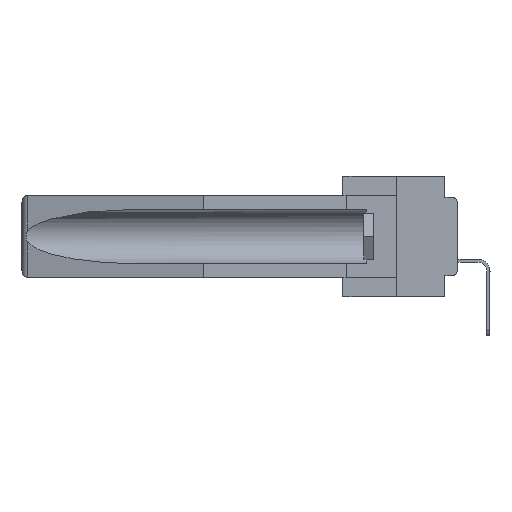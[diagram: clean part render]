
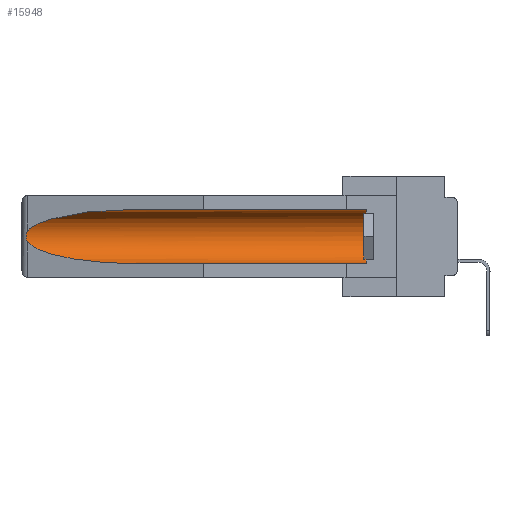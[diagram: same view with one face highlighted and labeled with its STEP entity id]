
A CAD part, left-side view. The second image highlights one B-rep face of the part: STEP entity #15948.
In plain terms, the highlighted cylindrical face has radius 2.857 mm (diameter 5.715 mm), a partial arc.
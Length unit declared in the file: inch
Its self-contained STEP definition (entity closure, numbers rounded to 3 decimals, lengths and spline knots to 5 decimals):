
#504 = B_SPLINE_CURVE_WITH_KNOTS ( 'NONE', 3,
 ( #11893, #12009, #11786, #32608, #19655, #22138, #32726, #30027, #14597, #22257 ),
 .UNSPECIFIED., .F., .F.,
 ( 4, 2, 2, 2, 4 ),
 ( 0., 0.00029, 0.00058, 0.00087, 0.00117 ),
 .UNSPECIFIED. ) ;
#1491 = CARTESIAN_POINT ( 'NONE',  ( 0.155, 0.126, -0.1715 ) ) ;
#1589 = CARTESIAN_POINT ( 'NONE',  ( 0.155, -0.30754, -0.1715 ) ) ;
#1916 = DIRECTION ( 'NONE',  ( 0., 0., 1. ) ) ;
#3488 = EDGE_CURVE ( 'NONE', #24629, #12277, #21368, .T. ) ;
#4004 = LINE ( 'NONE', #18733, #24552 ) ;
#4418 = CARTESIAN_POINT ( 'NONE',  ( 0.26537, 1.52718, -0.19328 ) ) ;
#4839 = AXIS2_PLACEMENT_3D ( 'NONE', #1491, #26967, #19302 ) ;
#5009 = AXIS2_PLACEMENT_3D ( 'NONE', #1589, #11741, #1916 ) ;
#5026 = EDGE_CURVE ( 'NONE', #12277, #6708, #504, .T. ) ;
#5242 = CARTESIAN_POINT ( 'NONE',  ( 0.21114, 1.30732, -0.284 ) ) ;
#6028 = CIRCLE ( 'NONE', #4839, 0.1125 ) ;
#6174 = EDGE_CURVE ( 'NONE', #6708, #15796, #25910, .T. ) ;
#6565 = CARTESIAN_POINT ( 'NONE',  ( 0.155, 1.07973, -0.284 ) ) ;
#6708 = VERTEX_POINT ( 'NONE', #4418 ) ;
#8124 = EDGE_LOOP ( 'NONE', ( #29429, #11922, #26573, #14606, #29176, #12643 ) ) ;
#8284 = CARTESIAN_POINT ( 'NONE',  ( 0.155, 1.07973, -0.059 ) ) ;
#10363 = CARTESIAN_POINT ( 'NONE',  ( 0.155, -0.30754, -0.059 ) ) ;
#11359 = CARTESIAN_POINT ( 'NONE',  ( 0.155, 1.07973, -0.059 ) ) ;
#11643 = VECTOR ( 'NONE', #31088, 39.37008 ) ;
#11741 = DIRECTION ( 'NONE',  ( 0., 1., 0. ) ) ;
#11786 = CARTESIAN_POINT ( 'NONE',  ( 0.26654, 1.53092, -0.15636 ) ) ;
#11893 = CARTESIAN_POINT ( 'NONE',  ( 0.26537, 1.52718, -0.14972 ) ) ;
#11922 = ORIENTED_EDGE ( 'NONE', *, *, #5026, .T. ) ;
#12009 = CARTESIAN_POINT ( 'NONE',  ( 0.26597, 1.52961, -0.15275 ) ) ;
#12277 = VERTEX_POINT ( 'NONE', #18742 ) ;
#12643 = ORIENTED_EDGE ( 'NONE', *, *, #25721, .T. ) ;
#13557 = DIRECTION ( 'NONE',  ( 0., 1., 0. ) ) ;
#14555 = CARTESIAN_POINT ( 'NONE',  ( 0.155, 0.126, -0.284 ) ) ;
#14597 = CARTESIAN_POINT ( 'NONE',  ( 0.26597, 1.5296, -0.19026 ) ) ;
#14606 = ORIENTED_EDGE ( 'NONE', *, *, #23876, .F. ) ;
#15796 = VERTEX_POINT ( 'NONE', #6565 ) ;
#15909 = VERTEX_POINT ( 'NONE', #14555 ) ;
#15948 = ADVANCED_FACE ( 'NONE', ( #29004 ), #29425, .F. ) ;
#16182 = CARTESIAN_POINT ( 'NONE',  ( 0.25451, 1.48313, -0.09465 ) ) ;
#16876 = LINE ( 'NONE', #10363, #11643 ) ;
#18733 = CARTESIAN_POINT ( 'NONE',  ( 0.155, -0.30754, -0.284 ) ) ;
#18742 = CARTESIAN_POINT ( 'NONE',  ( 0.26537, 1.52718, -0.14972 ) ) ;
#19302 = DIRECTION ( 'NONE',  ( 0., 0., 1. ) ) ;
#19655 = CARTESIAN_POINT ( 'NONE',  ( 0.2675, 1.53308, -0.16763 ) ) ;
#20410 = CARTESIAN_POINT ( 'NONE',  ( 0.155, 0.126, -0.059 ) ) ;
#21368 =( BOUNDED_CURVE ( )  B_SPLINE_CURVE ( 3, ( #8284, #26736, #16182, #26400 ),
 .UNSPECIFIED., .F., .F. ) 
 B_SPLINE_CURVE_WITH_KNOTS ( ( 4, 4 ),
 ( 4.71239, 6.08839 ),
 .UNSPECIFIED. ) 
 CURVE ( )  GEOMETRIC_REPRESENTATION_ITEM ( )  RATIONAL_B_SPLINE_CURVE ( ( 1., 0.848, 0.848, 1. ) ) 
 REPRESENTATION_ITEM ( '' )  );
#22138 = CARTESIAN_POINT ( 'NONE',  ( 0.2675, 1.53308, -0.17534 ) ) ;
#22257 = CARTESIAN_POINT ( 'NONE',  ( 0.26537, 1.52718, -0.19328 ) ) ;
#22937 = CARTESIAN_POINT ( 'NONE',  ( 0.155, 1.07973, -0.284 ) ) ;
#23876 = EDGE_CURVE ( 'NONE', #15909, #15796, #4004, .T. ) ;
#24552 = VECTOR ( 'NONE', #13557, 39.37008 ) ;
#24629 = VERTEX_POINT ( 'NONE', #11359 ) ;
#25721 = EDGE_CURVE ( 'NONE', #29948, #24629, #16876, .T. ) ;
#25910 =( BOUNDED_CURVE ( )  B_SPLINE_CURVE ( 3, ( #30817, #30926, #5242, #22937 ),
 .UNSPECIFIED., .F., .F. ) 
 B_SPLINE_CURVE_WITH_KNOTS ( ( 4, 4 ),
 ( 0.1948, 1.5708 ),
 .UNSPECIFIED. ) 
 CURVE ( )  GEOMETRIC_REPRESENTATION_ITEM ( )  RATIONAL_B_SPLINE_CURVE ( ( 1., 0.848, 0.848, 1. ) ) 
 REPRESENTATION_ITEM ( '' )  );
#26400 = CARTESIAN_POINT ( 'NONE',  ( 0.26537, 1.52718, -0.14972 ) ) ;
#26573 = ORIENTED_EDGE ( 'NONE', *, *, #6174, .T. ) ;
#26736 = CARTESIAN_POINT ( 'NONE',  ( 0.21114, 1.30732, -0.059 ) ) ;
#26967 = DIRECTION ( 'NONE',  ( 0., -1., 0. ) ) ;
#29004 = FACE_OUTER_BOUND ( 'NONE', #8124, .T. ) ;
#29176 = ORIENTED_EDGE ( 'NONE', *, *, #31408, .T. ) ;
#29425 = CYLINDRICAL_SURFACE ( 'NONE', #5009, 0.1125 ) ;
#29429 = ORIENTED_EDGE ( 'NONE', *, *, #3488, .T. ) ;
#29948 = VERTEX_POINT ( 'NONE', #20410 ) ;
#30027 = CARTESIAN_POINT ( 'NONE',  ( 0.26655, 1.53094, -0.18657 ) ) ;
#30817 = CARTESIAN_POINT ( 'NONE',  ( 0.26537, 1.52718, -0.19328 ) ) ;
#30926 = CARTESIAN_POINT ( 'NONE',  ( 0.25451, 1.48313, -0.24835 ) ) ;
#31088 = DIRECTION ( 'NONE',  ( 0., 1., 0. ) ) ;
#31408 = EDGE_CURVE ( 'NONE', #15909, #29948, #6028, .T. ) ;
#32608 = CARTESIAN_POINT ( 'NONE',  ( 0.2673, 1.5327, -0.16383 ) ) ;
#32726 = CARTESIAN_POINT ( 'NONE',  ( 0.2673, 1.53269, -0.17917 ) ) ;
